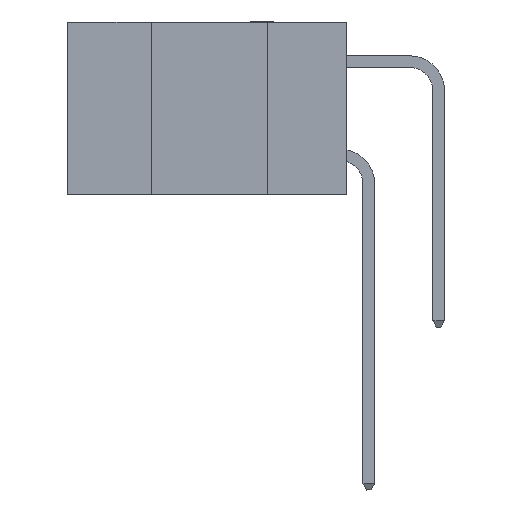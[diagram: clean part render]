
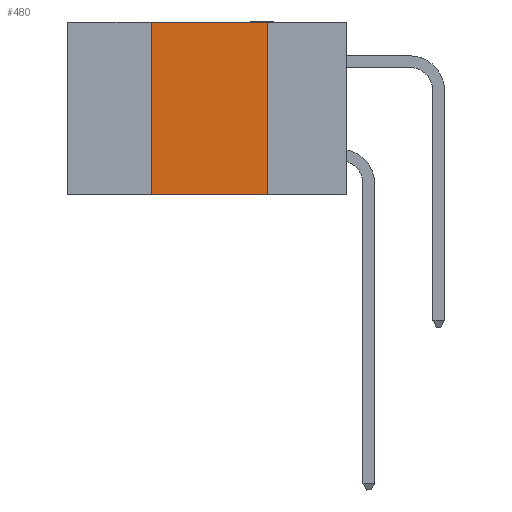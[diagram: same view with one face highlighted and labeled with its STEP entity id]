
A CAD part, left-side view. The second image highlights one B-rep face of the part: STEP entity #480.
In plain terms, the highlighted planar face has unit normal (-1, 0, 0).
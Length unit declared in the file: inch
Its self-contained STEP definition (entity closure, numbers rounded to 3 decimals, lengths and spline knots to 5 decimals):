
#104 = DIRECTION ( 'NONE',  ( 0., 0., -1. ) ) ;
#480 = ADVANCED_FACE ( 'NONE', ( #21751 ), #15634, .F. ) ;
#1053 = CARTESIAN_POINT ( 'NONE',  ( 0., 0.17, 0. ) ) ;
#2373 = DIRECTION ( 'NONE',  ( 0., 0., -1. ) ) ;
#5051 = DIRECTION ( 'NONE',  ( 1., 0., 0. ) ) ;
#5409 = CARTESIAN_POINT ( 'NONE',  ( 0., 0.42, -0.37 ) ) ;
#6618 = CARTESIAN_POINT ( 'NONE',  ( 0., 0.6, -0.37 ) ) ;
#7187 = ORIENTED_EDGE ( 'NONE', *, *, #37114, .F. ) ;
#7858 = VECTOR ( 'NONE', #38383, 39.37008 ) ;
#9505 = EDGE_CURVE ( 'NONE', #9667, #31941, #16756, .T. ) ;
#9667 = VERTEX_POINT ( 'NONE', #5409 ) ;
#10770 = EDGE_LOOP ( 'NONE', ( #7187, #39358, #12178, #15009 ) ) ;
#11187 = CARTESIAN_POINT ( 'NONE',  ( 0., 0.6, 0. ) ) ;
#12178 = ORIENTED_EDGE ( 'NONE', *, *, #9505, .F. ) ;
#14270 = DIRECTION ( 'NONE',  ( 0., -1., 0. ) ) ;
#15009 = ORIENTED_EDGE ( 'NONE', *, *, #15356, .T. ) ;
#15356 = EDGE_CURVE ( 'NONE', #9667, #15975, #28304, .T. ) ;
#15634 = PLANE ( 'NONE',  #40188 ) ;
#15975 = VERTEX_POINT ( 'NONE', #29454 ) ;
#16756 = LINE ( 'NONE', #22862, #7858 ) ;
#21751 = FACE_OUTER_BOUND ( 'NONE', #10770, .T. ) ;
#22343 = VERTEX_POINT ( 'NONE', #1053 ) ;
#22862 = CARTESIAN_POINT ( 'NONE',  ( 0., 0.42, 0. ) ) ;
#28304 = LINE ( 'NONE', #6618, #36219 ) ;
#29072 = VECTOR ( 'NONE', #104, 39.37008 ) ;
#29454 = CARTESIAN_POINT ( 'NONE',  ( 0., 0.17, -0.37 ) ) ;
#30946 = DIRECTION ( 'NONE',  ( 0., -1., 0. ) ) ;
#31621 = CARTESIAN_POINT ( 'NONE',  ( 0., 0.42, 0. ) ) ;
#31941 = VERTEX_POINT ( 'NONE', #31621 ) ;
#33973 = VECTOR ( 'NONE', #14270, 39.37008 ) ;
#34469 = LINE ( 'NONE', #38129, #29072 ) ;
#36219 = VECTOR ( 'NONE', #30946, 39.37008 ) ;
#36526 = CARTESIAN_POINT ( 'NONE',  ( 0., 0.6, 0. ) ) ;
#37114 = EDGE_CURVE ( 'NONE', #22343, #15975, #34469, .T. ) ;
#38129 = CARTESIAN_POINT ( 'NONE',  ( 0., 0.17, 0. ) ) ;
#38383 = DIRECTION ( 'NONE',  ( 0., 0., 1. ) ) ;
#38728 = EDGE_CURVE ( 'NONE', #31941, #22343, #39583, .T. ) ;
#39358 = ORIENTED_EDGE ( 'NONE', *, *, #38728, .F. ) ;
#39583 = LINE ( 'NONE', #11187, #33973 ) ;
#40188 = AXIS2_PLACEMENT_3D ( 'NONE', #36526, #5051, #2373 ) ;
